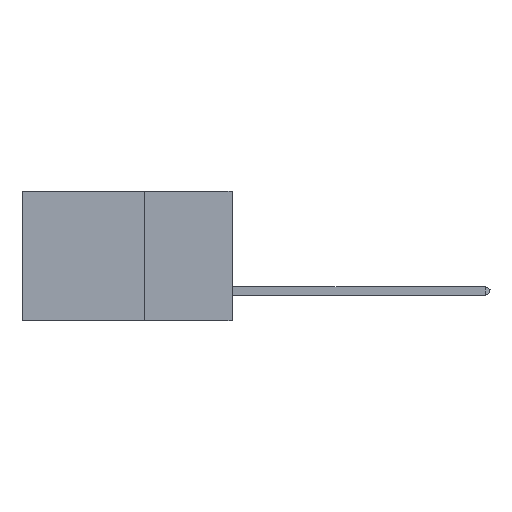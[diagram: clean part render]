
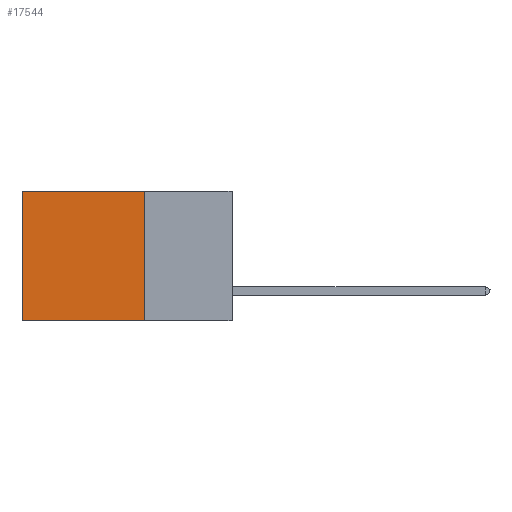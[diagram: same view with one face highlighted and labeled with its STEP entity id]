
A CAD part, left-side view. The second image highlights one B-rep face of the part: STEP entity #17544.
In plain terms, the highlighted planar face has unit normal (-1, 0, 0).
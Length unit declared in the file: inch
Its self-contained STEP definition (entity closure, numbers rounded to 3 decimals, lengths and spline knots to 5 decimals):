
#597 = CARTESIAN_POINT ( 'NONE',  ( 0.2875, 0.25, 0. ) ) ;
#1100 = CARTESIAN_POINT ( 'NONE',  ( 0.2875, 0.25, 0. ) ) ;
#1320 = CARTESIAN_POINT ( 'NONE',  ( 0.2875, 0.6, -0.37 ) ) ;
#3043 = CARTESIAN_POINT ( 'NONE',  ( 0.2875, 0.25, -0.37 ) ) ;
#3265 = EDGE_CURVE ( 'NONE', #19754, #7970, #5544, .T. ) ;
#4513 = FACE_OUTER_BOUND ( 'NONE', #6724, .T. ) ;
#4611 = LINE ( 'NONE', #6515, #18604 ) ;
#5333 = VECTOR ( 'NONE', #9027, 39.37008 ) ;
#5544 = LINE ( 'NONE', #25504, #14022 ) ;
#6515 = CARTESIAN_POINT ( 'NONE',  ( 0.2875, 0.25, 0. ) ) ;
#6724 = EDGE_LOOP ( 'NONE', ( #10280, #21938, #35031, #34272 ) ) ;
#7970 = VERTEX_POINT ( 'NONE', #1320 ) ;
#8798 = VECTOR ( 'NONE', #13744, 39.37008 ) ;
#8984 = DIRECTION ( 'NONE',  ( 0., 0., -1. ) ) ;
#9020 = VERTEX_POINT ( 'NONE', #3043 ) ;
#9027 = DIRECTION ( 'NONE',  ( 0., 1., 0. ) ) ;
#9189 = DIRECTION ( 'NONE',  ( 0., 0., -1. ) ) ;
#10280 = ORIENTED_EDGE ( 'NONE', *, *, #3265, .T. ) ;
#11799 = CARTESIAN_POINT ( 'NONE',  ( 0.2875, 0.6, 0. ) ) ;
#12648 = LINE ( 'NONE', #27274, #8798 ) ;
#13626 = VERTEX_POINT ( 'NONE', #597 ) ;
#13744 = DIRECTION ( 'NONE',  ( 0., 1., 0. ) ) ;
#14022 = VECTOR ( 'NONE', #9189, 39.37008 ) ;
#14717 = PLANE ( 'NONE',  #22390 ) ;
#17409 = DIRECTION ( 'NONE',  ( 1., 0., 0. ) ) ;
#17544 = ADVANCED_FACE ( 'NONE', ( #4513 ), #14717, .F. ) ;
#18578 = EDGE_CURVE ( 'NONE', #13626, #19754, #34199, .T. ) ;
#18604 = VECTOR ( 'NONE', #25548, 39.37008 ) ;
#19754 = VERTEX_POINT ( 'NONE', #11799 ) ;
#21938 = ORIENTED_EDGE ( 'NONE', *, *, #28937, .F. ) ;
#22390 = AXIS2_PLACEMENT_3D ( 'NONE', #25297, #17409, #8984 ) ;
#25297 = CARTESIAN_POINT ( 'NONE',  ( 0.2875, 0.25, 0. ) ) ;
#25504 = CARTESIAN_POINT ( 'NONE',  ( 0.2875, 0.6, 0. ) ) ;
#25548 = DIRECTION ( 'NONE',  ( 0., 0., -1. ) ) ;
#27274 = CARTESIAN_POINT ( 'NONE',  ( 0.2875, 0.25, -0.37 ) ) ;
#28528 = EDGE_CURVE ( 'NONE', #13626, #9020, #4611, .T. ) ;
#28937 = EDGE_CURVE ( 'NONE', #9020, #7970, #12648, .T. ) ;
#34199 = LINE ( 'NONE', #1100, #5333 ) ;
#34272 = ORIENTED_EDGE ( 'NONE', *, *, #18578, .T. ) ;
#35031 = ORIENTED_EDGE ( 'NONE', *, *, #28528, .F. ) ;
